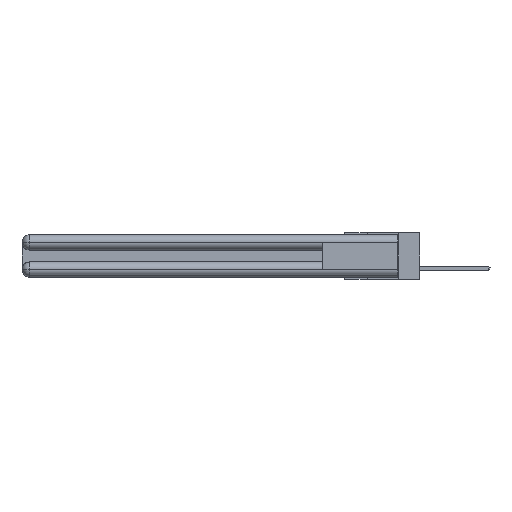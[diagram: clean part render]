
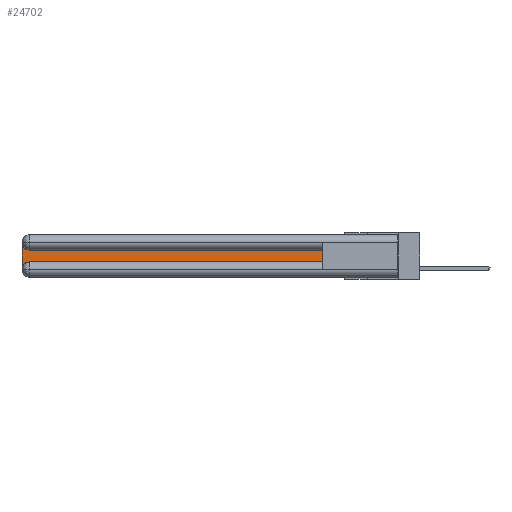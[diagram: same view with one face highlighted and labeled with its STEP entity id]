
A CAD part, left-side view. The second image highlights one B-rep face of the part: STEP entity #24702.
In plain terms, the highlighted planar face has unit normal (-1, 0, 0).
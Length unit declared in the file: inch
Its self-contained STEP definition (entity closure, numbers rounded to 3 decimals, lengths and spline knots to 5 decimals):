
#286 = DIRECTION ( 'NONE',  ( 0., 1., 0. ) ) ;
#394 = VERTEX_POINT ( 'NONE', #33418 ) ;
#1623 = ORIENTED_EDGE ( 'NONE', *, *, #8583, .T. ) ;
#2211 = EDGE_CURVE ( 'NONE', #11655, #17568, #23093, .T. ) ;
#2648 = DIRECTION ( 'NONE',  ( 1., 0., 0. ) ) ;
#4078 = EDGE_CURVE ( 'NONE', #16524, #11655, #30645, .T. ) ;
#5227 = DIRECTION ( 'NONE',  ( 0., 0., 1. ) ) ;
#6451 = DIRECTION ( 'NONE',  ( 0., 0., -1. ) ) ;
#6978 = CARTESIAN_POINT ( 'NONE',  ( 0.075, 0.6, -0.2175 ) ) ;
#7647 = CARTESIAN_POINT ( 'NONE',  ( 0.075, 2.94, -0.2175 ) ) ;
#7709 = CARTESIAN_POINT ( 'NONE',  ( 0.075, 3., -0.1225 ) ) ;
#7906 = VERTEX_POINT ( 'NONE', #25168 ) ;
#8140 = ORIENTED_EDGE ( 'NONE', *, *, #28489, .T. ) ;
#8583 = EDGE_CURVE ( 'NONE', #7906, #26073, #15002, .T. ) ;
#9013 = DIRECTION ( 'NONE',  ( 0., -1., 0. ) ) ;
#9927 = VECTOR ( 'NONE', #286, 39.37008 ) ;
#10305 = DIRECTION ( 'NONE',  ( 0., 0., -1. ) ) ;
#10379 = ORIENTED_EDGE ( 'NONE', *, *, #12482, .T. ) ;
#10564 = ORIENTED_EDGE ( 'NONE', *, *, #29853, .T. ) ;
#10593 = ORIENTED_EDGE ( 'NONE', *, *, #4078, .T. ) ;
#11655 = VERTEX_POINT ( 'NONE', #7647 ) ;
#12482 = EDGE_CURVE ( 'NONE', #394, #7906, #31743, .T. ) ;
#15002 = CIRCLE ( 'NONE', #31621, 0.06 ) ;
#15911 = CARTESIAN_POINT ( 'NONE',  ( 0.075, 2.94, -0.0625 ) ) ;
#16327 = AXIS2_PLACEMENT_3D ( 'NONE', #7709, #2648, #10305 ) ;
#16524 = VERTEX_POINT ( 'NONE', #20132 ) ;
#16826 = CARTESIAN_POINT ( 'NONE',  ( 0.075, 2.94, -0.2775 ) ) ;
#17568 = VERTEX_POINT ( 'NONE', #6978 ) ;
#17861 = LINE ( 'NONE', #32599, #27215 ) ;
#18504 = FACE_OUTER_BOUND ( 'NONE', #19738, .T. ) ;
#19738 = EDGE_LOOP ( 'NONE', ( #10379, #1623, #8140, #10593, #32422, #10564 ) ) ;
#20132 = CARTESIAN_POINT ( 'NONE',  ( 0.075, 3., -0.2775 ) ) ;
#20539 = CARTESIAN_POINT ( 'NONE',  ( 0.075, 0.6, -0.2175 ) ) ;
#20869 = DIRECTION ( 'NONE',  ( 0., 0., -1. ) ) ;
#21196 = DIRECTION ( 'NONE',  ( 1., 0., 0. ) ) ;
#23093 = LINE ( 'NONE', #24712, #27189 ) ;
#23583 = LINE ( 'NONE', #20539, #24379 ) ;
#24379 = VECTOR ( 'NONE', #5227, 39.37008 ) ;
#24702 = ADVANCED_FACE ( 'NONE', ( #18504 ), #33111, .F. ) ;
#24712 = CARTESIAN_POINT ( 'NONE',  ( 0.075, 0.6, -0.2175 ) ) ;
#25168 = CARTESIAN_POINT ( 'NONE',  ( 0.075, 2.94, -0.1225 ) ) ;
#25430 = CARTESIAN_POINT ( 'NONE',  ( 0.075, 3., -0.0625 ) ) ;
#26073 = VERTEX_POINT ( 'NONE', #25430 ) ;
#27189 = VECTOR ( 'NONE', #9013, 39.37008 ) ;
#27215 = VECTOR ( 'NONE', #29917, 39.37008 ) ;
#28489 = EDGE_CURVE ( 'NONE', #26073, #16524, #17861, .T. ) ;
#29619 = DIRECTION ( 'NONE',  ( 1., 0., 0. ) ) ;
#29853 = EDGE_CURVE ( 'NONE', #17568, #394, #23583, .T. ) ;
#29917 = DIRECTION ( 'NONE',  ( 0., 0., -1. ) ) ;
#30645 = CIRCLE ( 'NONE', #31320, 0.06 ) ;
#31176 = CARTESIAN_POINT ( 'NONE',  ( 0.075, 0.6, -0.1225 ) ) ;
#31320 = AXIS2_PLACEMENT_3D ( 'NONE', #16826, #29619, #6451 ) ;
#31621 = AXIS2_PLACEMENT_3D ( 'NONE', #15911, #21196, #20869 ) ;
#31743 = LINE ( 'NONE', #31176, #9927 ) ;
#32422 = ORIENTED_EDGE ( 'NONE', *, *, #2211, .T. ) ;
#32599 = CARTESIAN_POINT ( 'NONE',  ( 0.075, 3., -0.2175 ) ) ;
#33111 = PLANE ( 'NONE',  #16327 ) ;
#33418 = CARTESIAN_POINT ( 'NONE',  ( 0.075, 0.6, -0.1225 ) ) ;
